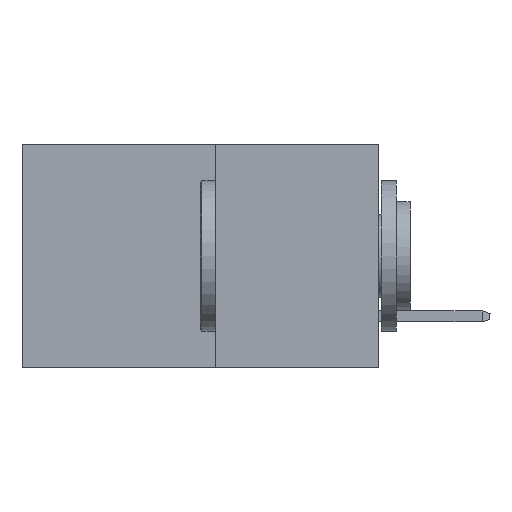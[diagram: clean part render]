
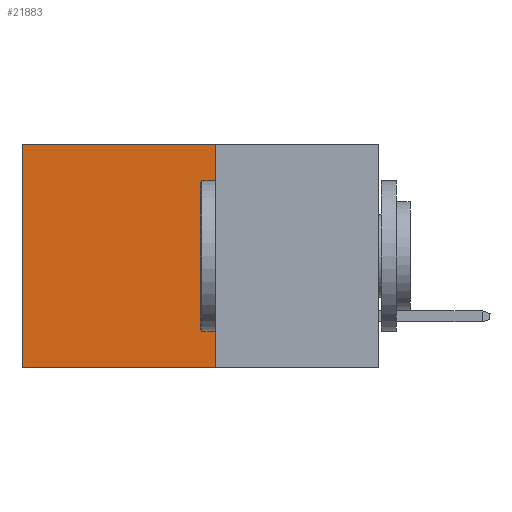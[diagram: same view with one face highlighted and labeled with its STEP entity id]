
A CAD part, left-side view. The second image highlights one B-rep face of the part: STEP entity #21883.
In plain terms, the highlighted planar face has unit normal (-1, 0, 0).
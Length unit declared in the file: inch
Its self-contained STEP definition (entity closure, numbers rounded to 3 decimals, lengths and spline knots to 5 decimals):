
#1050 = FACE_OUTER_BOUND ( 'NONE', #18060, .T. ) ;
#1132 = LINE ( 'NONE', #9886, #10266 ) ;
#2210 = EDGE_CURVE ( 'NONE', #19020, #4858, #22553, .T. ) ;
#2453 = ORIENTED_EDGE ( 'NONE', *, *, #2210, .F. ) ;
#2574 = DIRECTION ( 'NONE',  ( 0., 1., 0. ) ) ;
#2636 = DIRECTION ( 'NONE',  ( 0., 0., -1. ) ) ;
#3081 = VECTOR ( 'NONE', #19134, 39.37008 ) ;
#3688 = CARTESIAN_POINT ( 'NONE',  ( 0.277, 0.27, 0. ) ) ;
#4680 = CARTESIAN_POINT ( 'NONE',  ( 0.277, 0.59, 0. ) ) ;
#4858 = VERTEX_POINT ( 'NONE', #23217 ) ;
#5962 = ORIENTED_EDGE ( 'NONE', *, *, #9248, .T. ) ;
#6889 = VECTOR ( 'NONE', #21736, 39.37008 ) ;
#8185 = EDGE_CURVE ( 'NONE', #12382, #19020, #1132, .T. ) ;
#9248 = EDGE_CURVE ( 'NONE', #9910, #4858, #12751, .T. ) ;
#9400 = PLANE ( 'NONE',  #21133 ) ;
#9509 = CARTESIAN_POINT ( 'NONE',  ( 0.277, 0.27, -0.37 ) ) ;
#9886 = CARTESIAN_POINT ( 'NONE',  ( 0.277, 0.27, -0.37 ) ) ;
#9910 = VERTEX_POINT ( 'NONE', #4680 ) ;
#10266 = VECTOR ( 'NONE', #2636, 39.37008 ) ;
#10926 = CARTESIAN_POINT ( 'NONE',  ( 0.277, 0.27, 0. ) ) ;
#11292 = DIRECTION ( 'NONE',  ( 0., 0., -1. ) ) ;
#12247 = LINE ( 'NONE', #3688, #6889 ) ;
#12382 = VERTEX_POINT ( 'NONE', #10926 ) ;
#12751 = LINE ( 'NONE', #20870, #3081 ) ;
#12861 = ORIENTED_EDGE ( 'NONE', *, *, #14358, .T. ) ;
#14358 = EDGE_CURVE ( 'NONE', #12382, #9910, #12247, .T. ) ;
#14821 = CARTESIAN_POINT ( 'NONE',  ( 0.277, 0.27, -0.37 ) ) ;
#15381 = CARTESIAN_POINT ( 'NONE',  ( 0.277, 0.27, -0.37 ) ) ;
#18060 = EDGE_LOOP ( 'NONE', ( #5962, #2453, #20198, #12861 ) ) ;
#18968 = VECTOR ( 'NONE', #2574, 39.37008 ) ;
#19020 = VERTEX_POINT ( 'NONE', #15381 ) ;
#19134 = DIRECTION ( 'NONE',  ( 0., 0., -1. ) ) ;
#20198 = ORIENTED_EDGE ( 'NONE', *, *, #8185, .F. ) ;
#20870 = CARTESIAN_POINT ( 'NONE',  ( 0.277, 0.59, -0.37 ) ) ;
#21133 = AXIS2_PLACEMENT_3D ( 'NONE', #14821, #22019, #11292 ) ;
#21736 = DIRECTION ( 'NONE',  ( 0., 1., 0. ) ) ;
#21883 = ADVANCED_FACE ( 'NONE', ( #1050 ), #9400, .F. ) ;
#22019 = DIRECTION ( 'NONE',  ( 1., 0., 0. ) ) ;
#22553 = LINE ( 'NONE', #9509, #18968 ) ;
#23217 = CARTESIAN_POINT ( 'NONE',  ( 0.277, 0.59, -0.37 ) ) ;
